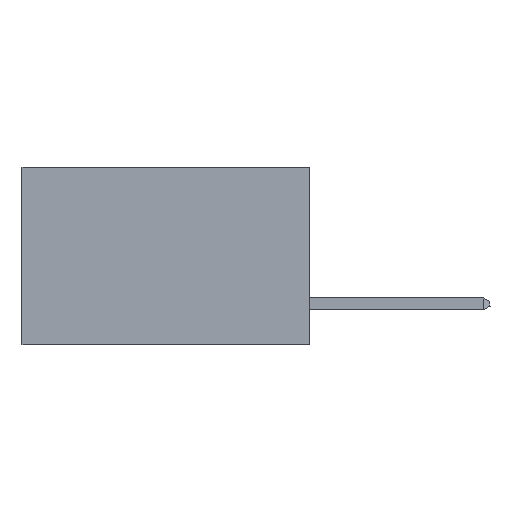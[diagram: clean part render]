
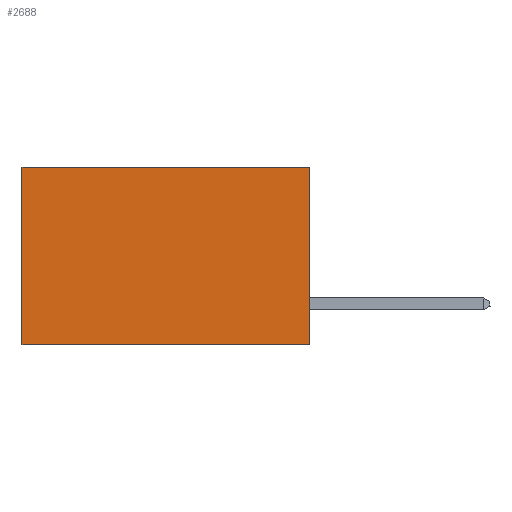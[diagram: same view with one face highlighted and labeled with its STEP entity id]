
A CAD part, left-side view. The second image highlights one B-rep face of the part: STEP entity #2688.
In plain terms, the highlighted planar face has unit normal (-1, 0, 0).
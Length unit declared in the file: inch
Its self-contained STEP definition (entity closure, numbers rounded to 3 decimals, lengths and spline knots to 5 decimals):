
#502 = DIRECTION ( 'NONE',  ( 1., 0., 0. ) ) ;
#1000 = DIRECTION ( 'NONE',  ( 0., 0., -1. ) ) ;
#1333 = EDGE_CURVE ( 'NONE', #2456, #10465, #5339, .T. ) ;
#1561 = VECTOR ( 'NONE', #5744, 39.37008 ) ;
#2127 = VECTOR ( 'NONE', #15412, 39.37008 ) ;
#2133 = DIRECTION ( 'NONE',  ( 0., 0., -1. ) ) ;
#2236 = ORIENTED_EDGE ( 'NONE', *, *, #9864, .T. ) ;
#2402 = CARTESIAN_POINT ( 'NONE',  ( 0.2875, 0., 0. ) ) ;
#2456 = VERTEX_POINT ( 'NONE', #6411 ) ;
#2688 = ADVANCED_FACE ( 'NONE', ( #13108 ), #7351, .F. ) ;
#2841 = EDGE_LOOP ( 'NONE', ( #4430, #16087, #11055, #2236 ) ) ;
#3050 = CARTESIAN_POINT ( 'NONE',  ( 0.2875, 0., 0. ) ) ;
#4430 = ORIENTED_EDGE ( 'NONE', *, *, #14434, .T. ) ;
#4733 = VECTOR ( 'NONE', #1000, 39.37008 ) ;
#5339 = LINE ( 'NONE', #2402, #4733 ) ;
#5744 = DIRECTION ( 'NONE',  ( 0., 0., -1. ) ) ;
#6253 = VERTEX_POINT ( 'NONE', #14197 ) ;
#6411 = CARTESIAN_POINT ( 'NONE',  ( 0.2875, 0., 0. ) ) ;
#6662 = DIRECTION ( 'NONE',  ( 0., 1., 0. ) ) ;
#6732 = CARTESIAN_POINT ( 'NONE',  ( 0.2875, 0., -0.37 ) ) ;
#6737 = CARTESIAN_POINT ( 'NONE',  ( 0.2875, 0.6, 0. ) ) ;
#7351 = PLANE ( 'NONE',  #11762 ) ;
#9054 = VERTEX_POINT ( 'NONE', #6737 ) ;
#9864 = EDGE_CURVE ( 'NONE', #2456, #9054, #13241, .T. ) ;
#10465 = VERTEX_POINT ( 'NONE', #6732 ) ;
#11055 = ORIENTED_EDGE ( 'NONE', *, *, #1333, .F. ) ;
#11058 = CARTESIAN_POINT ( 'NONE',  ( 0.2875, 0.6, 0. ) ) ;
#11762 = AXIS2_PLACEMENT_3D ( 'NONE', #3050, #502, #2133 ) ;
#13108 = FACE_OUTER_BOUND ( 'NONE', #2841, .T. ) ;
#13241 = LINE ( 'NONE', #14626, #15504 ) ;
#14197 = CARTESIAN_POINT ( 'NONE',  ( 0.2875, 0.6, -0.37 ) ) ;
#14434 = EDGE_CURVE ( 'NONE', #9054, #6253, #15434, .T. ) ;
#14626 = CARTESIAN_POINT ( 'NONE',  ( 0.2875, 0., 0. ) ) ;
#15351 = CARTESIAN_POINT ( 'NONE',  ( 0.2875, 0., -0.37 ) ) ;
#15412 = DIRECTION ( 'NONE',  ( 0., 1., 0. ) ) ;
#15434 = LINE ( 'NONE', #11058, #1561 ) ;
#15504 = VECTOR ( 'NONE', #6662, 39.37008 ) ;
#15965 = LINE ( 'NONE', #15351, #2127 ) ;
#16087 = ORIENTED_EDGE ( 'NONE', *, *, #16746, .F. ) ;
#16746 = EDGE_CURVE ( 'NONE', #10465, #6253, #15965, .T. ) ;
